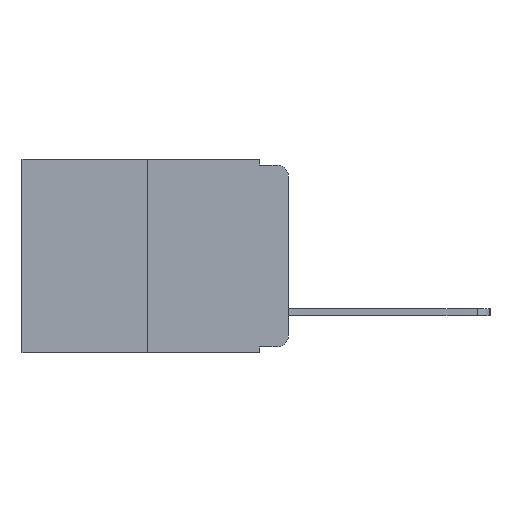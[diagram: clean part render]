
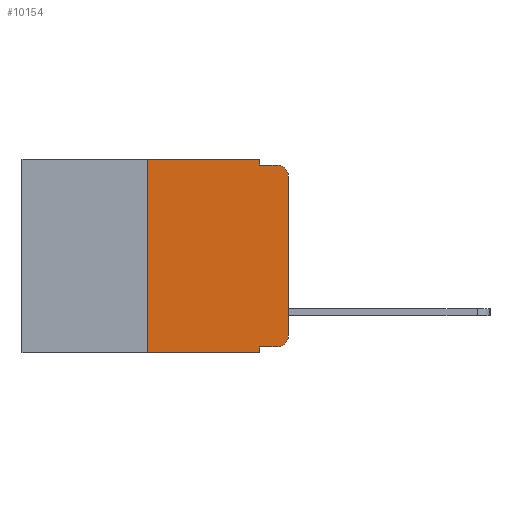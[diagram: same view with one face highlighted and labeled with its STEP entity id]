
A CAD part, left-side view. The second image highlights one B-rep face of the part: STEP entity #10154.
In plain terms, the highlighted planar face has unit normal (-1, 0, 0).
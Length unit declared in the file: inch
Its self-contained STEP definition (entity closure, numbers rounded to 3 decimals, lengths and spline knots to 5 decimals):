
#254 = VERTEX_POINT ( 'NONE', #1468 ) ;
#512 = CARTESIAN_POINT ( 'NONE',  ( 0., 0.051, 0. ) ) ;
#620 = VERTEX_POINT ( 'NONE', #6745 ) ;
#628 = VERTEX_POINT ( 'NONE', #18591 ) ;
#666 = CARTESIAN_POINT ( 'NONE',  ( 0., 0.051, -0.01 ) ) ;
#826 = VECTOR ( 'NONE', #17100, 39.37008 ) ;
#846 = EDGE_CURVE ( 'NONE', #2974, #6944, #5750, .T. ) ;
#939 = ORIENTED_EDGE ( 'NONE', *, *, #7123, .T. ) ;
#980 = VERTEX_POINT ( 'NONE', #17044 ) ;
#984 = ORIENTED_EDGE ( 'NONE', *, *, #7626, .T. ) ;
#1338 = ORIENTED_EDGE ( 'NONE', *, *, #16154, .F. ) ;
#1382 = ORIENTED_EDGE ( 'NONE', *, *, #16603, .F. ) ;
#1468 = CARTESIAN_POINT ( 'NONE',  ( 0., 0.051, -0.333 ) ) ;
#1586 = ORIENTED_EDGE ( 'NONE', *, *, #9384, .F. ) ;
#2091 = ORIENTED_EDGE ( 'NONE', *, *, #6215, .T. ) ;
#2114 = DIRECTION ( 'NONE',  ( -1., 0., 0. ) ) ;
#2119 = ORIENTED_EDGE ( 'NONE', *, *, #18914, .T. ) ;
#2221 = DIRECTION ( 'NONE',  ( 0., 0., -1. ) ) ;
#2725 = VERTEX_POINT ( 'NONE', #5010 ) ;
#2860 = ORIENTED_EDGE ( 'NONE', *, *, #16093, .F. ) ;
#2974 = VERTEX_POINT ( 'NONE', #16385 ) ;
#3476 = LINE ( 'NONE', #17702, #10864 ) ;
#3778 = ORIENTED_EDGE ( 'NONE', *, *, #846, .T. ) ;
#3918 = CARTESIAN_POINT ( 'NONE',  ( 0., 0.473, -0.343 ) ) ;
#4177 = CARTESIAN_POINT ( 'NONE',  ( 0., 0.02, -0.03 ) ) ;
#4332 = AXIS2_PLACEMENT_3D ( 'NONE', #13059, #4347, #14443 ) ;
#4347 = DIRECTION ( 'NONE',  ( 1., 0., 0. ) ) ;
#4468 = VECTOR ( 'NONE', #11420, 39.37008 ) ;
#4778 = VECTOR ( 'NONE', #18445, 39.37008 ) ;
#5010 = CARTESIAN_POINT ( 'NONE',  ( 0., 0.051, -0.343 ) ) ;
#5206 = CARTESIAN_POINT ( 'NONE',  ( 0., 0.051, 0. ) ) ;
#5555 = LINE ( 'NONE', #15762, #826 ) ;
#5653 = DIRECTION ( 'NONE',  ( 0., 0., -1. ) ) ;
#5750 = CIRCLE ( 'NONE', #15518, 0.02 ) ;
#6153 = VECTOR ( 'NONE', #13859, 39.37008 ) ;
#6215 = EDGE_CURVE ( 'NONE', #620, #2725, #13074, .T. ) ;
#6521 = VERTEX_POINT ( 'NONE', #11805 ) ;
#6626 = LINE ( 'NONE', #512, #14275 ) ;
#6745 = CARTESIAN_POINT ( 'NONE',  ( 0., 0.25, -0.343 ) ) ;
#6944 = VERTEX_POINT ( 'NONE', #18195 ) ;
#7123 = EDGE_CURVE ( 'NONE', #6521, #10598, #15606, .T. ) ;
#7626 = EDGE_CURVE ( 'NONE', #6944, #6521, #5555, .T. ) ;
#7954 = DIRECTION ( 'NONE',  ( 0., 0., 1. ) ) ;
#9222 = LINE ( 'NONE', #10295, #4778 ) ;
#9384 = EDGE_CURVE ( 'NONE', #628, #13405, #9222, .T. ) ;
#9892 = DIRECTION ( 'NONE',  ( 0., -1., 0. ) ) ;
#9921 = CARTESIAN_POINT ( 'NONE',  ( 0., 0.051, -0.333 ) ) ;
#10122 = DIRECTION ( 'NONE',  ( 0., -1., 0. ) ) ;
#10154 = ADVANCED_FACE ( 'NONE', ( #18654 ), #11666, .F. ) ;
#10295 = CARTESIAN_POINT ( 'NONE',  ( 0., 0.473, 0. ) ) ;
#10359 = AXIS2_PLACEMENT_3D ( 'NONE', #4177, #14279, #5653 ) ;
#10506 = EDGE_LOOP ( 'NONE', ( #984, #939, #1338, #1382, #1586, #16809, #2091, #2860, #2119, #3778 ) ) ;
#10598 = VERTEX_POINT ( 'NONE', #15201 ) ;
#10864 = VECTOR ( 'NONE', #7954, 39.37008 ) ;
#11420 = DIRECTION ( 'NONE',  ( 0., -1., 0. ) ) ;
#11666 = PLANE ( 'NONE',  #4332 ) ;
#11805 = CARTESIAN_POINT ( 'NONE',  ( 0., 0., -0.03 ) ) ;
#12548 = VECTOR ( 'NONE', #9892, 39.37008 ) ;
#13059 = CARTESIAN_POINT ( 'NONE',  ( 0., 0.473, 0. ) ) ;
#13074 = LINE ( 'NONE', #3918, #15848 ) ;
#13219 = EDGE_CURVE ( 'NONE', #620, #628, #3476, .T. ) ;
#13405 = VERTEX_POINT ( 'NONE', #18055 ) ;
#13834 = LINE ( 'NONE', #5206, #6153 ) ;
#13859 = DIRECTION ( 'NONE',  ( 0., 0., -1. ) ) ;
#14275 = VECTOR ( 'NONE', #2221, 39.37008 ) ;
#14279 = DIRECTION ( 'NONE',  ( -1., 0., 0. ) ) ;
#14443 = DIRECTION ( 'NONE',  ( 0., 0., -1. ) ) ;
#15201 = CARTESIAN_POINT ( 'NONE',  ( 0., 0.02, -0.01 ) ) ;
#15518 = AXIS2_PLACEMENT_3D ( 'NONE', #17063, #2114, #17690 ) ;
#15606 = CIRCLE ( 'NONE', #10359, 0.02 ) ;
#15762 = CARTESIAN_POINT ( 'NONE',  ( 0., 0., 0. ) ) ;
#15848 = VECTOR ( 'NONE', #10122, 39.37008 ) ;
#15889 = LINE ( 'NONE', #9921, #4468 ) ;
#16093 = EDGE_CURVE ( 'NONE', #254, #2725, #6626, .T. ) ;
#16154 = EDGE_CURVE ( 'NONE', #980, #10598, #16592, .T. ) ;
#16385 = CARTESIAN_POINT ( 'NONE',  ( 0., 0.02, -0.333 ) ) ;
#16592 = LINE ( 'NONE', #666, #12548 ) ;
#16603 = EDGE_CURVE ( 'NONE', #13405, #980, #13834, .T. ) ;
#16809 = ORIENTED_EDGE ( 'NONE', *, *, #13219, .F. ) ;
#17044 = CARTESIAN_POINT ( 'NONE',  ( 0., 0.051, -0.01 ) ) ;
#17063 = CARTESIAN_POINT ( 'NONE',  ( 0., 0.02, -0.313 ) ) ;
#17100 = DIRECTION ( 'NONE',  ( 0., 0., 1. ) ) ;
#17690 = DIRECTION ( 'NONE',  ( 0., 0., -1. ) ) ;
#17702 = CARTESIAN_POINT ( 'NONE',  ( 0., 0.25, 0. ) ) ;
#18055 = CARTESIAN_POINT ( 'NONE',  ( 0., 0.051, 0. ) ) ;
#18195 = CARTESIAN_POINT ( 'NONE',  ( 0., 0., -0.313 ) ) ;
#18445 = DIRECTION ( 'NONE',  ( 0., -1., 0. ) ) ;
#18591 = CARTESIAN_POINT ( 'NONE',  ( 0., 0.25, 0. ) ) ;
#18654 = FACE_OUTER_BOUND ( 'NONE', #10506, .T. ) ;
#18914 = EDGE_CURVE ( 'NONE', #254, #2974, #15889, .T. ) ;
